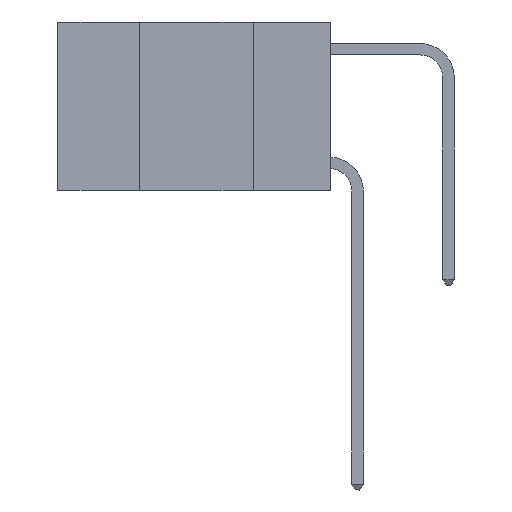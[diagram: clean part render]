
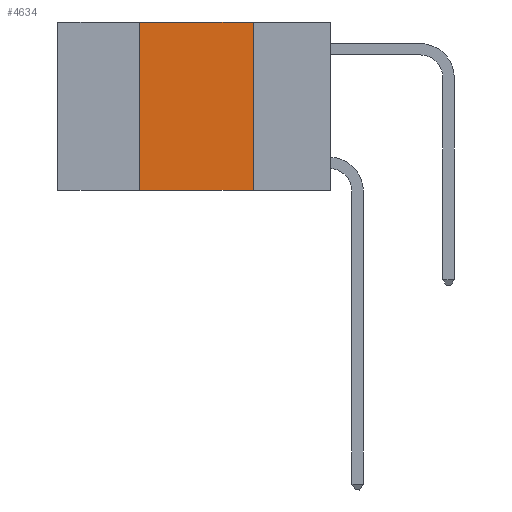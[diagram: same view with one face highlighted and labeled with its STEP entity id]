
A CAD part, left-side view. The second image highlights one B-rep face of the part: STEP entity #4634.
In plain terms, the highlighted planar face has unit normal (-1, 0, 0).
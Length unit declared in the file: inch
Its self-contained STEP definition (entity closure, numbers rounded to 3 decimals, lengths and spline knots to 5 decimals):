
#385 = EDGE_CURVE ( 'NONE', #3177, #12549, #11806, .T. ) ;
#457 = DIRECTION ( 'NONE',  ( 0., -1., 0. ) ) ;
#858 = ORIENTED_EDGE ( 'NONE', *, *, #7192, .F. ) ;
#1030 = VERTEX_POINT ( 'NONE', #4335 ) ;
#1385 = LINE ( 'NONE', #12613, #2300 ) ;
#1698 = ORIENTED_EDGE ( 'NONE', *, *, #8199, .F. ) ;
#1727 = ORIENTED_EDGE ( 'NONE', *, *, #4313, .T. ) ;
#2300 = VECTOR ( 'NONE', #10077, 39.37008 ) ;
#2535 = LINE ( 'NONE', #9440, #6405 ) ;
#3177 = VERTEX_POINT ( 'NONE', #11667 ) ;
#3259 = LINE ( 'NONE', #7333, #12370 ) ;
#3466 = AXIS2_PLACEMENT_3D ( 'NONE', #12333, #10518, #4597 ) ;
#4313 = EDGE_CURVE ( 'NONE', #3177, #1030, #2535, .T. ) ;
#4335 = CARTESIAN_POINT ( 'NONE',  ( 0., 0.17, -0.37 ) ) ;
#4597 = DIRECTION ( 'NONE',  ( 0., 0., -1. ) ) ;
#4634 = ADVANCED_FACE ( 'NONE', ( #11471 ), #5425, .F. ) ;
#4698 = CARTESIAN_POINT ( 'NONE',  ( 0., 0.17, 0. ) ) ;
#5425 = PLANE ( 'NONE',  #3466 ) ;
#6405 = VECTOR ( 'NONE', #8311, 39.37008 ) ;
#6620 = CARTESIAN_POINT ( 'NONE',  ( 0., 0.42, 0. ) ) ;
#7192 = EDGE_CURVE ( 'NONE', #10850, #1030, #1385, .T. ) ;
#7333 = CARTESIAN_POINT ( 'NONE',  ( 0., 0.6, 0. ) ) ;
#7452 = CARTESIAN_POINT ( 'NONE',  ( 0., 0.42, 0. ) ) ;
#8121 = VECTOR ( 'NONE', #10212, 39.37008 ) ;
#8199 = EDGE_CURVE ( 'NONE', #12549, #10850, #3259, .T. ) ;
#8311 = DIRECTION ( 'NONE',  ( 0., -1., 0. ) ) ;
#9440 = CARTESIAN_POINT ( 'NONE',  ( 0., 0.6, -0.37 ) ) ;
#9555 = ORIENTED_EDGE ( 'NONE', *, *, #385, .F. ) ;
#10077 = DIRECTION ( 'NONE',  ( 0., 0., -1. ) ) ;
#10212 = DIRECTION ( 'NONE',  ( 0., 0., 1. ) ) ;
#10407 = EDGE_LOOP ( 'NONE', ( #858, #1698, #9555, #1727 ) ) ;
#10518 = DIRECTION ( 'NONE',  ( 1., 0., 0. ) ) ;
#10850 = VERTEX_POINT ( 'NONE', #4698 ) ;
#11471 = FACE_OUTER_BOUND ( 'NONE', #10407, .T. ) ;
#11667 = CARTESIAN_POINT ( 'NONE',  ( 0., 0.42, -0.37 ) ) ;
#11806 = LINE ( 'NONE', #6620, #8121 ) ;
#12333 = CARTESIAN_POINT ( 'NONE',  ( 0., 0.6, 0. ) ) ;
#12370 = VECTOR ( 'NONE', #457, 39.37008 ) ;
#12549 = VERTEX_POINT ( 'NONE', #7452 ) ;
#12613 = CARTESIAN_POINT ( 'NONE',  ( 0., 0.17, 0. ) ) ;
